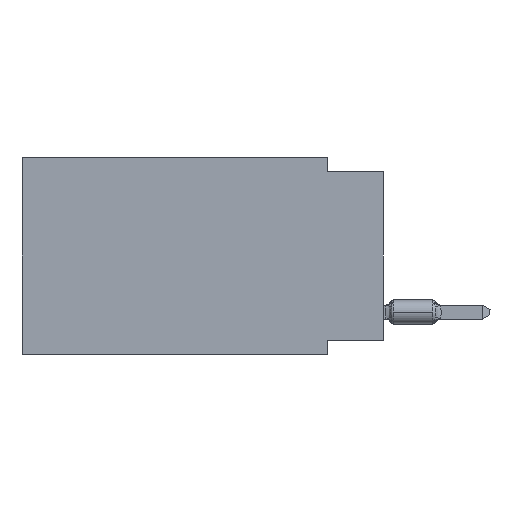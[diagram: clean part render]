
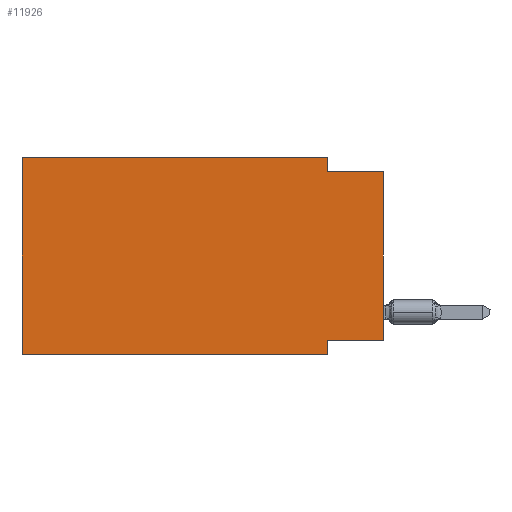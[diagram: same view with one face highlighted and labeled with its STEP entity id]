
A CAD part, left-side view. The second image highlights one B-rep face of the part: STEP entity #11926.
In plain terms, the highlighted planar face has unit normal (-1, 0, 0).
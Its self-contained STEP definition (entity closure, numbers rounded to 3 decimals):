
#597 = DIRECTION ( 'NONE',  ( 1., 0., 0. ) ) ;
#667 = CARTESIAN_POINT ( 'NONE',  ( 0., 16.383, 0. ) ) ;
#1005 = CARTESIAN_POINT ( 'NONE',  ( 0., 2.54, -8.89 ) ) ;
#1164 = CARTESIAN_POINT ( 'NONE',  ( 0., 0., -8.255 ) ) ;
#1342 = AXIS2_PLACEMENT_3D ( 'NONE', #8534, #597, #38820 ) ;
#1632 = CARTESIAN_POINT ( 'NONE',  ( 0., 0., -8.255 ) ) ;
#4642 = ORIENTED_EDGE ( 'NONE', *, *, #34404, .F. ) ;
#7146 = CARTESIAN_POINT ( 'NONE',  ( 0., 2.54, -8.89 ) ) ;
#7273 = VERTEX_POINT ( 'NONE', #38609 ) ;
#7279 = VERTEX_POINT ( 'NONE', #22797 ) ;
#7786 = VERTEX_POINT ( 'NONE', #48449 ) ;
#8534 = CARTESIAN_POINT ( 'NONE',  ( 0., 16.383, 0. ) ) ;
#8818 = CARTESIAN_POINT ( 'NONE',  ( 0., 16.383, 0. ) ) ;
#9536 = DIRECTION ( 'NONE',  ( 0., 0., 1. ) ) ;
#11332 = ORIENTED_EDGE ( 'NONE', *, *, #41442, .F. ) ;
#11433 = EDGE_CURVE ( 'NONE', #38302, #7786, #49172, .T. ) ;
#11926 = ADVANCED_FACE ( 'NONE', ( #28556 ), #44654, .F. ) ;
#13502 = CARTESIAN_POINT ( 'NONE',  ( 0., 0., 0. ) ) ;
#16245 = EDGE_CURVE ( 'NONE', #25973, #23584, #33523, .T. ) ;
#17324 = VERTEX_POINT ( 'NONE', #29056 ) ;
#19233 = LINE ( 'NONE', #23715, #20705 ) ;
#20705 = VECTOR ( 'NONE', #34819, 1000. ) ;
#21524 = LINE ( 'NONE', #37629, #38333 ) ;
#22039 = ORIENTED_EDGE ( 'NONE', *, *, #48632, .F. ) ;
#22797 = CARTESIAN_POINT ( 'NONE',  ( 0., 2.54, -8.255 ) ) ;
#23221 = DIRECTION ( 'NONE',  ( 0., 0., -1. ) ) ;
#23584 = VERTEX_POINT ( 'NONE', #42407 ) ;
#23715 = CARTESIAN_POINT ( 'NONE',  ( 0., 2.54, 0. ) ) ;
#23944 = CARTESIAN_POINT ( 'NONE',  ( 0., 0., -0.635 ) ) ;
#25287 = VECTOR ( 'NONE', #28864, 1000. ) ;
#25417 = DIRECTION ( 'NONE',  ( 0., 1., 0. ) ) ;
#25936 = LINE ( 'NONE', #8818, #25287 ) ;
#25973 = VERTEX_POINT ( 'NONE', #1632 ) ;
#28173 = ORIENTED_EDGE ( 'NONE', *, *, #44844, .F. ) ;
#28556 = FACE_OUTER_BOUND ( 'NONE', #31066, .T. ) ;
#28864 = DIRECTION ( 'NONE',  ( 0., -1., 0. ) ) ;
#29056 = CARTESIAN_POINT ( 'NONE',  ( 0., 2.54, 0. ) ) ;
#30073 = ORIENTED_EDGE ( 'NONE', *, *, #16245, .T. ) ;
#31066 = EDGE_LOOP ( 'NONE', ( #30073, #11332, #4642, #28173, #46065, #38656, #22039, #47754 ) ) ;
#31503 = VECTOR ( 'NONE', #23221, 1000. ) ;
#33523 = LINE ( 'NONE', #13502, #34423 ) ;
#34404 = EDGE_CURVE ( 'NONE', #17324, #7273, #19233, .T. ) ;
#34423 = VECTOR ( 'NONE', #9536, 1000. ) ;
#34819 = DIRECTION ( 'NONE',  ( 0., 0., -1. ) ) ;
#35579 = VERTEX_POINT ( 'NONE', #1005 ) ;
#36029 = CARTESIAN_POINT ( 'NONE',  ( 0., 16.383, -8.89 ) ) ;
#37629 = CARTESIAN_POINT ( 'NONE',  ( 0., 16.383, -8.89 ) ) ;
#38302 = VERTEX_POINT ( 'NONE', #36029 ) ;
#38333 = VECTOR ( 'NONE', #41840, 1000. ) ;
#38609 = CARTESIAN_POINT ( 'NONE',  ( 0., 2.54, -0.635 ) ) ;
#38656 = ORIENTED_EDGE ( 'NONE', *, *, #47581, .T. ) ;
#38820 = DIRECTION ( 'NONE',  ( 0., 0., -1. ) ) ;
#38823 = LINE ( 'NONE', #23944, #40317 ) ;
#40317 = VECTOR ( 'NONE', #47073, 1000. ) ;
#41442 = EDGE_CURVE ( 'NONE', #7273, #23584, #38823, .T. ) ;
#41840 = DIRECTION ( 'NONE',  ( 0., -1., 0. ) ) ;
#42407 = CARTESIAN_POINT ( 'NONE',  ( 0., 0., -0.635 ) ) ;
#44654 = PLANE ( 'NONE',  #1342 ) ;
#44844 = EDGE_CURVE ( 'NONE', #7786, #17324, #25936, .T. ) ;
#44940 = LINE ( 'NONE', #1164, #50291 ) ;
#45751 = DIRECTION ( 'NONE',  ( 0., 0., 1. ) ) ;
#45948 = VECTOR ( 'NONE', #45751, 1000. ) ;
#46065 = ORIENTED_EDGE ( 'NONE', *, *, #11433, .F. ) ;
#47073 = DIRECTION ( 'NONE',  ( 0., -1., 0. ) ) ;
#47581 = EDGE_CURVE ( 'NONE', #38302, #35579, #21524, .T. ) ;
#47754 = ORIENTED_EDGE ( 'NONE', *, *, #51450, .F. ) ;
#48449 = CARTESIAN_POINT ( 'NONE',  ( 0., 16.383, 0. ) ) ;
#48632 = EDGE_CURVE ( 'NONE', #7279, #35579, #51193, .T. ) ;
#49172 = LINE ( 'NONE', #667, #45948 ) ;
#50291 = VECTOR ( 'NONE', #25417, 1000. ) ;
#51193 = LINE ( 'NONE', #7146, #31503 ) ;
#51450 = EDGE_CURVE ( 'NONE', #25973, #7279, #44940, .T. ) ;
